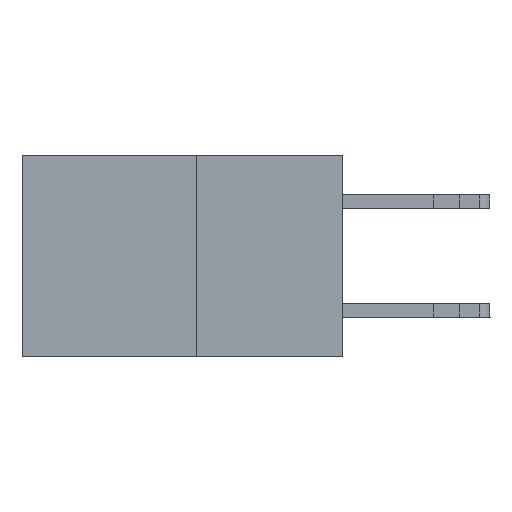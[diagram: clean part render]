
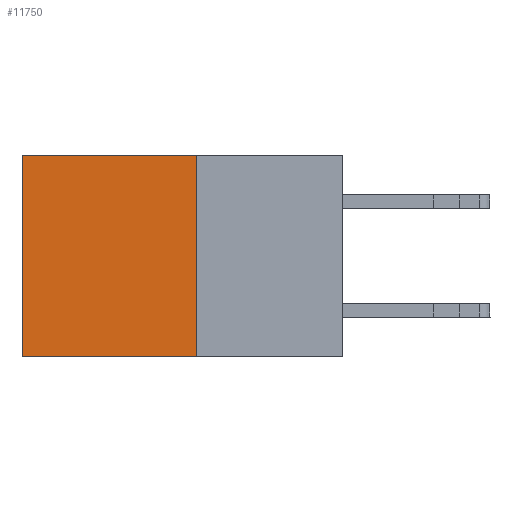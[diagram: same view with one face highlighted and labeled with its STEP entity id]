
A CAD part, left-side view. The second image highlights one B-rep face of the part: STEP entity #11750.
In plain terms, the highlighted planar face has unit normal (-1, 0, 0).
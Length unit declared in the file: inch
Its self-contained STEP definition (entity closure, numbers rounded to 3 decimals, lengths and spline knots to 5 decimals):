
#14 = CARTESIAN_POINT ( 'NONE',  ( 0.277, 0.59, -0.37 ) ) ;
#786 = DIRECTION ( 'NONE',  ( 1., 0., 0. ) ) ;
#903 = ORIENTED_EDGE ( 'NONE', *, *, #17674, .T. ) ;
#2125 = DIRECTION ( 'NONE',  ( 0., 0., -1. ) ) ;
#3117 = EDGE_CURVE ( 'NONE', #21882, #7237, #8488, .T. ) ;
#7237 = VERTEX_POINT ( 'NONE', #14 ) ;
#7512 = EDGE_LOOP ( 'NONE', ( #13514, #11172, #15468, #903 ) ) ;
#7627 = VECTOR ( 'NONE', #10908, 39.37008 ) ;
#8003 = LINE ( 'NONE', #13457, #23672 ) ;
#8230 = AXIS2_PLACEMENT_3D ( 'NONE', #10215, #786, #14032 ) ;
#8241 = CARTESIAN_POINT ( 'NONE',  ( 0.277, 0.27, -0.37 ) ) ;
#8488 = LINE ( 'NONE', #11290, #14155 ) ;
#8979 = CARTESIAN_POINT ( 'NONE',  ( 0.277, 0.27, 0. ) ) ;
#10215 = CARTESIAN_POINT ( 'NONE',  ( 0.277, 0.27, -0.37 ) ) ;
#10908 = DIRECTION ( 'NONE',  ( 0., 1., 0. ) ) ;
#11035 = EDGE_CURVE ( 'NONE', #21101, #7237, #13951, .T. ) ;
#11148 = DIRECTION ( 'NONE',  ( 0., 0., -1. ) ) ;
#11172 = ORIENTED_EDGE ( 'NONE', *, *, #11035, .F. ) ;
#11290 = CARTESIAN_POINT ( 'NONE',  ( 0.277, 0.59, -0.37 ) ) ;
#11605 = DIRECTION ( 'NONE',  ( 0., 1., 0. ) ) ;
#11750 = ADVANCED_FACE ( 'NONE', ( #17999 ), #23385, .F. ) ;
#13457 = CARTESIAN_POINT ( 'NONE',  ( 0.277, 0.27, -0.37 ) ) ;
#13514 = ORIENTED_EDGE ( 'NONE', *, *, #3117, .T. ) ;
#13951 = LINE ( 'NONE', #22872, #15107 ) ;
#14032 = DIRECTION ( 'NONE',  ( 0., 0., -1. ) ) ;
#14155 = VECTOR ( 'NONE', #11148, 39.37008 ) ;
#15107 = VECTOR ( 'NONE', #11605, 39.37008 ) ;
#15468 = ORIENTED_EDGE ( 'NONE', *, *, #20814, .F. ) ;
#17585 = CARTESIAN_POINT ( 'NONE',  ( 0.277, 0.27, 0. ) ) ;
#17674 = EDGE_CURVE ( 'NONE', #19568, #21882, #22701, .T. ) ;
#17950 = CARTESIAN_POINT ( 'NONE',  ( 0.277, 0.59, 0. ) ) ;
#17999 = FACE_OUTER_BOUND ( 'NONE', #7512, .T. ) ;
#19568 = VERTEX_POINT ( 'NONE', #17585 ) ;
#20814 = EDGE_CURVE ( 'NONE', #19568, #21101, #8003, .T. ) ;
#21101 = VERTEX_POINT ( 'NONE', #8241 ) ;
#21882 = VERTEX_POINT ( 'NONE', #17950 ) ;
#22701 = LINE ( 'NONE', #8979, #7627 ) ;
#22872 = CARTESIAN_POINT ( 'NONE',  ( 0.277, 0.27, -0.37 ) ) ;
#23385 = PLANE ( 'NONE',  #8230 ) ;
#23672 = VECTOR ( 'NONE', #2125, 39.37008 ) ;
